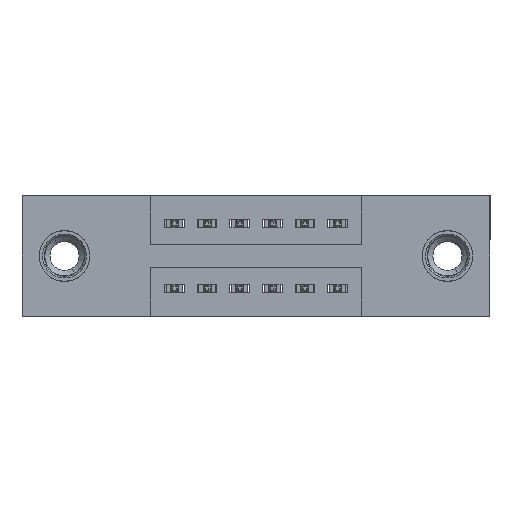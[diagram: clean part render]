
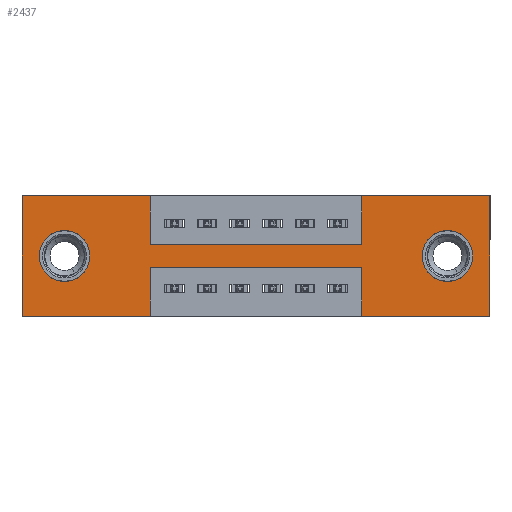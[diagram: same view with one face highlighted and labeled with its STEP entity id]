
A CAD part, front view. The second image highlights one B-rep face of the part: STEP entity #2437.
In plain terms, the highlighted planar face has unit normal (0, -1, 0).
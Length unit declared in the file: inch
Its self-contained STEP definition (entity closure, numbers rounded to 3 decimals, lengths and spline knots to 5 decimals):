
#53 = VERTEX_POINT ( 'NONE', #2240 ) ;
#167 = AXIS2_PLACEMENT_3D ( 'NONE', #1200, #9226, #3742 ) ;
#237 = CIRCLE ( 'NONE', #1883, 0.078 ) ;
#603 = LINE ( 'NONE', #9356, #9764 ) ;
#613 = EDGE_CURVE ( 'NONE', #4012, #10118, #9416, .T. ) ;
#620 = CARTESIAN_POINT ( 'NONE',  ( 1.0425, 0., 0. ) ) ;
#805 = FACE_BOUND ( 'NONE', #2613, .T. ) ;
#832 = CARTESIAN_POINT ( 'NONE',  ( 1.0425, 0., -0.37 ) ) ;
#886 = CARTESIAN_POINT ( 'NONE',  ( 0.3925, 0., 0. ) ) ;
#891 = VECTOR ( 'NONE', #11725, 39.37008 ) ;
#1024 = DIRECTION ( 'NONE',  ( 1., 0., 0. ) ) ;
#1185 = EDGE_CURVE ( 'NONE', #7088, #5110, #237, .T. ) ;
#1200 = CARTESIAN_POINT ( 'NONE',  ( 0.13, 0., -0.185 ) ) ;
#1421 = CARTESIAN_POINT ( 'NONE',  ( 1.0425, 0., -0.37 ) ) ;
#1468 = VECTOR ( 'NONE', #1750, 39.37008 ) ;
#1680 = EDGE_CURVE ( 'NONE', #11069, #4012, #4901, .T. ) ;
#1748 = LINE ( 'NONE', #886, #891 ) ;
#1750 = DIRECTION ( 'NONE',  ( 0., 0., 1. ) ) ;
#1846 = CARTESIAN_POINT ( 'NONE',  ( 0., 0., 0. ) ) ;
#1883 = AXIS2_PLACEMENT_3D ( 'NONE', #9517, #4027, #9394 ) ;
#1893 = EDGE_CURVE ( 'NONE', #4430, #5055, #603, .T. ) ;
#1900 = CARTESIAN_POINT ( 'NONE',  ( 0., 0., -0.37 ) ) ;
#1919 = ORIENTED_EDGE ( 'NONE', *, *, #1185, .T. ) ;
#1944 = EDGE_CURVE ( 'NONE', #5110, #7088, #4003, .T. ) ;
#1955 = CARTESIAN_POINT ( 'NONE',  ( 0.3925, 0., -0.22 ) ) ;
#2051 = CIRCLE ( 'NONE', #3883, 0.078 ) ;
#2169 = LINE ( 'NONE', #4926, #10341 ) ;
#2240 = CARTESIAN_POINT ( 'NONE',  ( 1.305, 0., -0.107 ) ) ;
#2331 = DIRECTION ( 'NONE',  ( -1., 0., 0. ) ) ;
#2437 = ADVANCED_FACE ( 'NONE', ( #7402, #805, #3394 ), #10141, .T. ) ;
#2599 = VECTOR ( 'NONE', #8218, 39.37008 ) ;
#2613 = EDGE_LOOP ( 'NONE', ( #11547, #1919 ) ) ;
#2714 = CARTESIAN_POINT ( 'NONE',  ( 0.3925, 0., -0.15 ) ) ;
#2721 = LINE ( 'NONE', #2948, #9023 ) ;
#2751 = ORIENTED_EDGE ( 'NONE', *, *, #613, .F. ) ;
#2818 = VERTEX_POINT ( 'NONE', #6822 ) ;
#2940 = EDGE_CURVE ( 'NONE', #9884, #4701, #1748, .T. ) ;
#2948 = CARTESIAN_POINT ( 'NONE',  ( 0., 0., 0. ) ) ;
#3109 = ORIENTED_EDGE ( 'NONE', *, *, #10073, .F. ) ;
#3116 = VECTOR ( 'NONE', #5867, 39.37008 ) ;
#3196 = AXIS2_PLACEMENT_3D ( 'NONE', #1900, #4694, #7269 ) ;
#3281 = DIRECTION ( 'NONE',  ( 0., 1., 0. ) ) ;
#3394 = FACE_OUTER_BOUND ( 'NONE', #10521, .T. ) ;
#3610 = VERTEX_POINT ( 'NONE', #1846 ) ;
#3628 = DIRECTION ( 'NONE',  ( 0., 0., 1. ) ) ;
#3742 = DIRECTION ( 'NONE',  ( 0., 0., 1. ) ) ;
#3780 = VECTOR ( 'NONE', #7535, 39.37008 ) ;
#3832 = ORIENTED_EDGE ( 'NONE', *, *, #5740, .F. ) ;
#3883 = AXIS2_PLACEMENT_3D ( 'NONE', #11518, #3281, #5000 ) ;
#3930 = LINE ( 'NONE', #5765, #3780 ) ;
#4003 = CIRCLE ( 'NONE', #167, 0.078 ) ;
#4012 = VERTEX_POINT ( 'NONE', #7729 ) ;
#4020 = LINE ( 'NONE', #7978, #6600 ) ;
#4027 = DIRECTION ( 'NONE',  ( 0., 1., 0. ) ) ;
#4049 = ORIENTED_EDGE ( 'NONE', *, *, #9102, .F. ) ;
#4430 = VERTEX_POINT ( 'NONE', #620 ) ;
#4490 = EDGE_CURVE ( 'NONE', #6337, #53, #2051, .T. ) ;
#4505 = LINE ( 'NONE', #9112, #11531 ) ;
#4690 = EDGE_CURVE ( 'NONE', #9106, #4430, #4505, .T. ) ;
#4694 = DIRECTION ( 'NONE',  ( 0., -1., 0. ) ) ;
#4701 = VERTEX_POINT ( 'NONE', #2714 ) ;
#4786 = DIRECTION ( 'NONE',  ( 0., 0., 1. ) ) ;
#4788 = CARTESIAN_POINT ( 'NONE',  ( 0., 0., -0.37 ) ) ;
#4901 = LINE ( 'NONE', #832, #1468 ) ;
#4926 = CARTESIAN_POINT ( 'NONE',  ( 1.435, 0., 0. ) ) ;
#4973 = VERTEX_POINT ( 'NONE', #5828 ) ;
#5000 = DIRECTION ( 'NONE',  ( 0., 0., -1. ) ) ;
#5055 = VERTEX_POINT ( 'NONE', #6967 ) ;
#5110 = VERTEX_POINT ( 'NONE', #7584 ) ;
#5200 = CARTESIAN_POINT ( 'NONE',  ( 0.13, 0., -0.263 ) ) ;
#5206 = ORIENTED_EDGE ( 'NONE', *, *, #4490, .T. ) ;
#5519 = VECTOR ( 'NONE', #7718, 39.37008 ) ;
#5740 = EDGE_CURVE ( 'NONE', #4701, #9106, #3930, .T. ) ;
#5765 = CARTESIAN_POINT ( 'NONE',  ( 0.3925, 0., -0.15 ) ) ;
#5828 = CARTESIAN_POINT ( 'NONE',  ( 1.435, 0., -0.37 ) ) ;
#5867 = DIRECTION ( 'NONE',  ( 1., 0., 0. ) ) ;
#5904 = EDGE_CURVE ( 'NONE', #4973, #11069, #9809, .T. ) ;
#6071 = CARTESIAN_POINT ( 'NONE',  ( 1.305, 0., -0.185 ) ) ;
#6284 = ORIENTED_EDGE ( 'NONE', *, *, #9995, .F. ) ;
#6285 = VERTEX_POINT ( 'NONE', #4788 ) ;
#6337 = VERTEX_POINT ( 'NONE', #11271 ) ;
#6338 = DIRECTION ( 'NONE',  ( 0., 0., -1. ) ) ;
#6350 = VECTOR ( 'NONE', #2331, 39.37008 ) ;
#6408 = LINE ( 'NONE', #6752, #3116 ) ;
#6600 = VECTOR ( 'NONE', #6338, 39.37008 ) ;
#6601 = CARTESIAN_POINT ( 'NONE',  ( 0.3925, 0., -0.22 ) ) ;
#6752 = CARTESIAN_POINT ( 'NONE',  ( 0., 0., 0. ) ) ;
#6822 = CARTESIAN_POINT ( 'NONE',  ( 0.3925, 0., -0.37 ) ) ;
#6893 = LINE ( 'NONE', #8108, #2599 ) ;
#6966 = DIRECTION ( 'NONE',  ( 0., 1., 0. ) ) ;
#6967 = CARTESIAN_POINT ( 'NONE',  ( 1.435, 0., 0. ) ) ;
#7000 = DIRECTION ( 'NONE',  ( 0., 0., -1. ) ) ;
#7088 = VERTEX_POINT ( 'NONE', #5200 ) ;
#7227 = ORIENTED_EDGE ( 'NONE', *, *, #1680, .F. ) ;
#7259 = AXIS2_PLACEMENT_3D ( 'NONE', #6071, #6966, #7000 ) ;
#7269 = DIRECTION ( 'NONE',  ( 0., 0., -1. ) ) ;
#7402 = FACE_BOUND ( 'NONE', #10104, .T. ) ;
#7535 = DIRECTION ( 'NONE',  ( 1., 0., 0. ) ) ;
#7564 = ORIENTED_EDGE ( 'NONE', *, *, #4690, .F. ) ;
#7584 = CARTESIAN_POINT ( 'NONE',  ( 0.13, 0., -0.107 ) ) ;
#7718 = DIRECTION ( 'NONE',  ( -1., 0., 0. ) ) ;
#7729 = CARTESIAN_POINT ( 'NONE',  ( 1.0425, 0., -0.22 ) ) ;
#7978 = CARTESIAN_POINT ( 'NONE',  ( 0.3925, 0., -0.37 ) ) ;
#8108 = CARTESIAN_POINT ( 'NONE',  ( 0., 0., -0.37 ) ) ;
#8150 = CARTESIAN_POINT ( 'NONE',  ( 0.3925, 0., 0. ) ) ;
#8218 = DIRECTION ( 'NONE',  ( -1., 0., 0. ) ) ;
#8355 = ORIENTED_EDGE ( 'NONE', *, *, #9019, .F. ) ;
#8520 = CARTESIAN_POINT ( 'NONE',  ( 1.0425, 0., -0.15 ) ) ;
#8602 = CARTESIAN_POINT ( 'NONE',  ( 0., 0., -0.37 ) ) ;
#8867 = CIRCLE ( 'NONE', #7259, 0.078 ) ;
#9019 = EDGE_CURVE ( 'NONE', #10118, #2818, #4020, .T. ) ;
#9023 = VECTOR ( 'NONE', #4786, 39.37008 ) ;
#9102 = EDGE_CURVE ( 'NONE', #5055, #4973, #2169, .T. ) ;
#9106 = VERTEX_POINT ( 'NONE', #8520 ) ;
#9112 = CARTESIAN_POINT ( 'NONE',  ( 1.0425, 0., 0. ) ) ;
#9226 = DIRECTION ( 'NONE',  ( 0., 1., 0. ) ) ;
#9267 = ORIENTED_EDGE ( 'NONE', *, *, #10396, .T. ) ;
#9279 = ORIENTED_EDGE ( 'NONE', *, *, #5904, .F. ) ;
#9356 = CARTESIAN_POINT ( 'NONE',  ( 0., 0., 0. ) ) ;
#9394 = DIRECTION ( 'NONE',  ( 0., 0., 1. ) ) ;
#9416 = LINE ( 'NONE', #6601, #5519 ) ;
#9517 = CARTESIAN_POINT ( 'NONE',  ( 0.13, 0., -0.185 ) ) ;
#9539 = DIRECTION ( 'NONE',  ( 0., 0., -1. ) ) ;
#9627 = ORIENTED_EDGE ( 'NONE', *, *, #11135, .F. ) ;
#9764 = VECTOR ( 'NONE', #1024, 39.37008 ) ;
#9809 = LINE ( 'NONE', #8602, #6350 ) ;
#9884 = VERTEX_POINT ( 'NONE', #8150 ) ;
#9995 = EDGE_CURVE ( 'NONE', #2818, #6285, #6893, .T. ) ;
#10073 = EDGE_CURVE ( 'NONE', #6285, #3610, #2721, .T. ) ;
#10104 = EDGE_LOOP ( 'NONE', ( #9267, #5206 ) ) ;
#10118 = VERTEX_POINT ( 'NONE', #1955 ) ;
#10141 = PLANE ( 'NONE',  #3196 ) ;
#10341 = VECTOR ( 'NONE', #9539, 39.37008 ) ;
#10396 = EDGE_CURVE ( 'NONE', #53, #6337, #8867, .T. ) ;
#10521 = EDGE_LOOP ( 'NONE', ( #8355, #2751, #7227, #9279, #4049, #11190, #7564, #3832, #11159, #9627, #3109, #6284 ) ) ;
#11069 = VERTEX_POINT ( 'NONE', #1421 ) ;
#11135 = EDGE_CURVE ( 'NONE', #3610, #9884, #6408, .T. ) ;
#11159 = ORIENTED_EDGE ( 'NONE', *, *, #2940, .F. ) ;
#11190 = ORIENTED_EDGE ( 'NONE', *, *, #1893, .F. ) ;
#11271 = CARTESIAN_POINT ( 'NONE',  ( 1.305, 0., -0.263 ) ) ;
#11518 = CARTESIAN_POINT ( 'NONE',  ( 1.305, 0., -0.185 ) ) ;
#11531 = VECTOR ( 'NONE', #3628, 39.37008 ) ;
#11547 = ORIENTED_EDGE ( 'NONE', *, *, #1944, .T. ) ;
#11725 = DIRECTION ( 'NONE',  ( 0., 0., -1. ) ) ;
